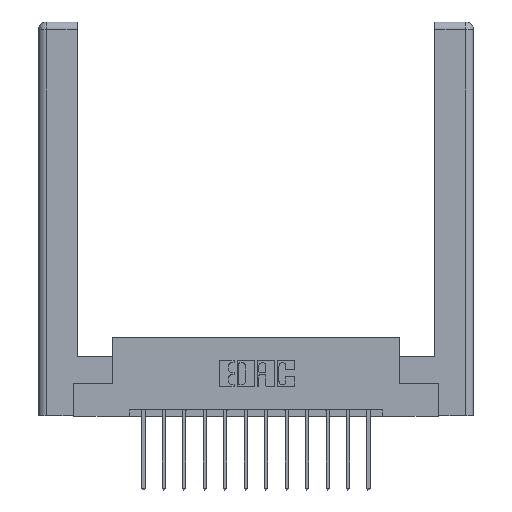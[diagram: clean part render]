
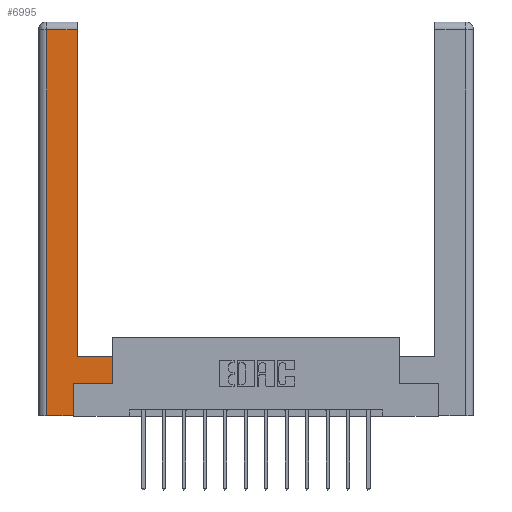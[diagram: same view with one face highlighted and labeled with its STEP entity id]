
A CAD part, top view. The second image highlights one B-rep face of the part: STEP entity #6995.
In plain terms, the highlighted planar face has unit normal (0, 0, 1).
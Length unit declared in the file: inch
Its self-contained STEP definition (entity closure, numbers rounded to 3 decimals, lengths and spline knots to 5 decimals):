
#222 = ORIENTED_EDGE ( 'NONE', *, *, #11242, .T. ) ;
#251 = VERTEX_POINT ( 'NONE', #1469 ) ;
#375 = CARTESIAN_POINT ( 'NONE',  ( 0., 0., 0. ) ) ;
#472 = DIRECTION ( 'NONE',  ( 0., 1., 0. ) ) ;
#480 = DIRECTION ( 'NONE',  ( 0., 1., 0. ) ) ;
#591 = VECTOR ( 'NONE', #8133, 39.37008 ) ;
#707 = ORIENTED_EDGE ( 'NONE', *, *, #2118, .T. ) ;
#1058 = LINE ( 'NONE', #1961, #11568 ) ;
#1384 = EDGE_CURVE ( 'NONE', #12677, #3904, #1432, .T. ) ;
#1432 = LINE ( 'NONE', #14099, #13636 ) ;
#1469 = CARTESIAN_POINT ( 'NONE',  ( 0.265, 0.245, 0. ) ) ;
#1576 = DIRECTION ( 'NONE',  ( 1., 0., 0. ) ) ;
#1814 = VECTOR ( 'NONE', #480, 39.37008 ) ;
#1820 = VERTEX_POINT ( 'NONE', #14692 ) ;
#1961 = CARTESIAN_POINT ( 'NONE',  ( 0.295, 0.45, 0. ) ) ;
#2025 = CARTESIAN_POINT ( 'NONE',  ( 0.565, 0.245, 0. ) ) ;
#2118 = EDGE_CURVE ( 'NONE', #3904, #251, #7543, .T. ) ;
#2516 = ORIENTED_EDGE ( 'NONE', *, *, #1384, .T. ) ;
#2733 = DIRECTION ( 'NONE',  ( -1., 0., 0. ) ) ;
#2895 = CARTESIAN_POINT ( 'NONE',  ( 0.295, 3., 0. ) ) ;
#2925 = DIRECTION ( 'NONE',  ( 0., -1., 0. ) ) ;
#3558 = EDGE_CURVE ( 'NONE', #11587, #1820, #10162, .T. ) ;
#3904 = VERTEX_POINT ( 'NONE', #12801 ) ;
#4391 = DIRECTION ( 'NONE',  ( 0., 1., 0. ) ) ;
#4599 = VECTOR ( 'NONE', #472, 39.37008 ) ;
#4905 = CARTESIAN_POINT ( 'NONE',  ( 0.0615, 2.94, 0. ) ) ;
#5746 = LINE ( 'NONE', #9032, #10951 ) ;
#5904 = VECTOR ( 'NONE', #10894, 39.37008 ) ;
#6296 = PLANE ( 'NONE',  #13690 ) ;
#6432 = ORIENTED_EDGE ( 'NONE', *, *, #7711, .T. ) ;
#6585 = FACE_OUTER_BOUND ( 'NONE', #10813, .T. ) ;
#6995 = ADVANCED_FACE ( 'NONE', ( #6585 ), #6296, .F. ) ;
#7543 = LINE ( 'NONE', #15394, #12123 ) ;
#7711 = EDGE_CURVE ( 'NONE', #251, #11587, #11112, .T. ) ;
#7774 = EDGE_CURVE ( 'NONE', #14240, #13664, #9580, .T. ) ;
#8133 = DIRECTION ( 'NONE',  ( 1., 0., 0. ) ) ;
#8993 = DIRECTION ( 'NONE',  ( -1., 0., 0. ) ) ;
#9032 = CARTESIAN_POINT ( 'NONE',  ( 0.0615, 0., 0. ) ) ;
#9217 = ORIENTED_EDGE ( 'NONE', *, *, #3558, .T. ) ;
#9580 = LINE ( 'NONE', #4905, #5904 ) ;
#9905 = CARTESIAN_POINT ( 'NONE',  ( 0.565, 0.245, 0. ) ) ;
#10104 = CARTESIAN_POINT ( 'NONE',  ( 0.295, 2.94, 0. ) ) ;
#10162 = LINE ( 'NONE', #12657, #4599 ) ;
#10374 = ORIENTED_EDGE ( 'NONE', *, *, #11291, .T. ) ;
#10813 = EDGE_LOOP ( 'NONE', ( #222, #12569, #12336, #2516, #707, #6432, #9217, #10374 ) ) ;
#10894 = DIRECTION ( 'NONE',  ( -1., 0., 0. ) ) ;
#10951 = VECTOR ( 'NONE', #2925, 39.37008 ) ;
#11051 = CARTESIAN_POINT ( 'NONE',  ( 0.295, 0.45, 0. ) ) ;
#11112 = LINE ( 'NONE', #2025, #591 ) ;
#11242 = EDGE_CURVE ( 'NONE', #15053, #14240, #12523, .T. ) ;
#11285 = DIRECTION ( 'NONE',  ( 0., 0., -1. ) ) ;
#11291 = EDGE_CURVE ( 'NONE', #1820, #15053, #1058, .T. ) ;
#11568 = VECTOR ( 'NONE', #8993, 39.37008 ) ;
#11587 = VERTEX_POINT ( 'NONE', #9905 ) ;
#12123 = VECTOR ( 'NONE', #4391, 39.37008 ) ;
#12336 = ORIENTED_EDGE ( 'NONE', *, *, #13067, .T. ) ;
#12523 = LINE ( 'NONE', #2895, #1814 ) ;
#12569 = ORIENTED_EDGE ( 'NONE', *, *, #7774, .T. ) ;
#12657 = CARTESIAN_POINT ( 'NONE',  ( 0.565, 0.45, 0. ) ) ;
#12677 = VERTEX_POINT ( 'NONE', #13940 ) ;
#12801 = CARTESIAN_POINT ( 'NONE',  ( 0.265, 0., 0. ) ) ;
#13067 = EDGE_CURVE ( 'NONE', #13664, #12677, #5746, .T. ) ;
#13480 = CARTESIAN_POINT ( 'NONE',  ( 0.0615, 2.94, 0. ) ) ;
#13636 = VECTOR ( 'NONE', #1576, 39.37008 ) ;
#13664 = VERTEX_POINT ( 'NONE', #13480 ) ;
#13690 = AXIS2_PLACEMENT_3D ( 'NONE', #375, #11285, #2733 ) ;
#13940 = CARTESIAN_POINT ( 'NONE',  ( 0.0615, 0., 0. ) ) ;
#14099 = CARTESIAN_POINT ( 'NONE',  ( 0.265, 0., 0. ) ) ;
#14240 = VERTEX_POINT ( 'NONE', #10104 ) ;
#14692 = CARTESIAN_POINT ( 'NONE',  ( 0.565, 0.45, 0. ) ) ;
#15053 = VERTEX_POINT ( 'NONE', #11051 ) ;
#15394 = CARTESIAN_POINT ( 'NONE',  ( 0.265, 0.245, 0. ) ) ;
